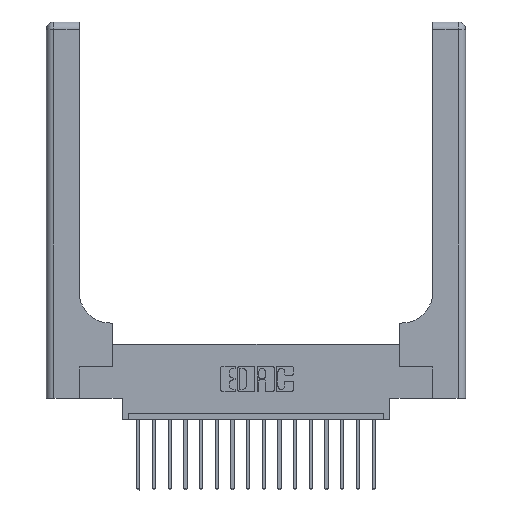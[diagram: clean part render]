
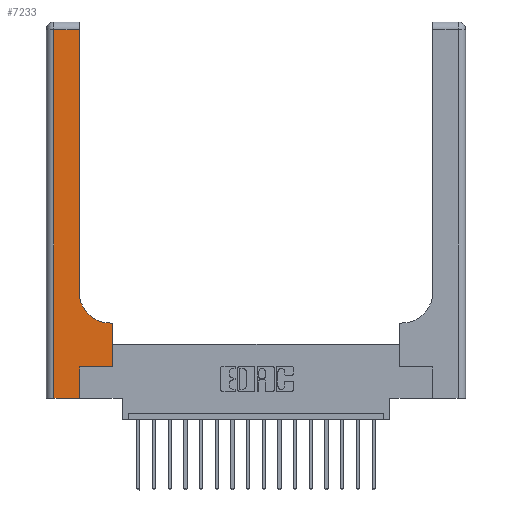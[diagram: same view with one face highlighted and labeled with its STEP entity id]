
A CAD part, top view. The second image highlights one B-rep face of the part: STEP entity #7233.
In plain terms, the highlighted planar face has unit normal (0, 0, 1).
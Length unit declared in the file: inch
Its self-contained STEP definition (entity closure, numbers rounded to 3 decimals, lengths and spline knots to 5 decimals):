
#9 = CARTESIAN_POINT ( 'NONE',  ( 0.06, 3., 0.37 ) ) ;
#205 = LINE ( 'NONE', #4086, #1102 ) ;
#412 = ORIENTED_EDGE ( 'NONE', *, *, #15414, .T. ) ;
#486 = DIRECTION ( 'NONE',  ( -1., 0., 0. ) ) ;
#812 = VECTOR ( 'NONE', #4106, 39.37008 ) ;
#978 = EDGE_LOOP ( 'NONE', ( #1641, #412, #14996, #4080, #8999, #10588, #2637, #17993, #13572 ) ) ;
#985 = CARTESIAN_POINT ( 'NONE',  ( 0., 2.94, 0.37 ) ) ;
#1102 = VECTOR ( 'NONE', #8644, 39.37008 ) ;
#1524 = CARTESIAN_POINT ( 'NONE',  ( 0., 0., 0.37 ) ) ;
#1550 = VECTOR ( 'NONE', #486, 39.37008 ) ;
#1641 = ORIENTED_EDGE ( 'NONE', *, *, #18540, .T. ) ;
#1730 = VERTEX_POINT ( 'NONE', #8140 ) ;
#2637 = ORIENTED_EDGE ( 'NONE', *, *, #5337, .T. ) ;
#2975 = VECTOR ( 'NONE', #3086, 39.37008 ) ;
#3002 = VECTOR ( 'NONE', #10304, 39.37008 ) ;
#3086 = DIRECTION ( 'NONE',  ( 0., -1., 0. ) ) ;
#3801 = DIRECTION ( 'NONE',  ( -1., 0., 0. ) ) ;
#3985 = CARTESIAN_POINT ( 'NONE',  ( 0.51, 0.6, 0.37 ) ) ;
#4080 = ORIENTED_EDGE ( 'NONE', *, *, #17657, .T. ) ;
#4086 = CARTESIAN_POINT ( 'NONE',  ( 0.26, 3., 0.37 ) ) ;
#4106 = DIRECTION ( 'NONE',  ( 1., 0., 0. ) ) ;
#4174 = LINE ( 'NONE', #18143, #18634 ) ;
#5337 = EDGE_CURVE ( 'NONE', #13479, #11984, #10361, .T. ) ;
#5340 = DIRECTION ( 'NONE',  ( 1., 0., 0. ) ) ;
#5829 = VECTOR ( 'NONE', #3801, 39.37008 ) ;
#6020 = CARTESIAN_POINT ( 'NONE',  ( 0.26, 2.94, 0.37 ) ) ;
#6306 = LINE ( 'NONE', #8536, #812 ) ;
#6322 = LINE ( 'NONE', #12239, #1550 ) ;
#6421 = VERTEX_POINT ( 'NONE', #3985 ) ;
#6530 = DIRECTION ( 'NONE',  ( 0., 0., -1. ) ) ;
#6581 = VERTEX_POINT ( 'NONE', #17558 ) ;
#6830 = LINE ( 'NONE', #9, #2975 ) ;
#7233 = ADVANCED_FACE ( 'NONE', ( #8741 ), #17638, .F. ) ;
#8039 = CARTESIAN_POINT ( 'NONE',  ( 0., 3., 0.37 ) ) ;
#8140 = CARTESIAN_POINT ( 'NONE',  ( 0.265, 0., 0.37 ) ) ;
#8175 = CIRCLE ( 'NONE', #14443, 0.25 ) ;
#8536 = CARTESIAN_POINT ( 'NONE',  ( 0.265, 0.25, 0.37 ) ) ;
#8644 = DIRECTION ( 'NONE',  ( 0., 1., 0. ) ) ;
#8741 = FACE_OUTER_BOUND ( 'NONE', #978, .T. ) ;
#8908 = AXIS2_PLACEMENT_3D ( 'NONE', #8039, #9368, #10792 ) ;
#8999 = ORIENTED_EDGE ( 'NONE', *, *, #17158, .T. ) ;
#9368 = DIRECTION ( 'NONE',  ( 0., 0., -1. ) ) ;
#9685 = LINE ( 'NONE', #985, #5829 ) ;
#9704 = VECTOR ( 'NONE', #17058, 39.37008 ) ;
#10067 = CARTESIAN_POINT ( 'NONE',  ( 0.265, 0.25, 0.37 ) ) ;
#10304 = DIRECTION ( 'NONE',  ( 1., 0., 0. ) ) ;
#10361 = LINE ( 'NONE', #12723, #9704 ) ;
#10588 = ORIENTED_EDGE ( 'NONE', *, *, #13125, .T. ) ;
#10792 = DIRECTION ( 'NONE',  ( -1., 0., 0. ) ) ;
#10891 = DIRECTION ( 'NONE',  ( 0., 1., 0. ) ) ;
#11281 = VERTEX_POINT ( 'NONE', #18059 ) ;
#11462 = CARTESIAN_POINT ( 'NONE',  ( 0.06, 2.94, 0.37 ) ) ;
#11984 = VERTEX_POINT ( 'NONE', #15474 ) ;
#12239 = CARTESIAN_POINT ( 'NONE',  ( 0.26, 0.6, 0.37 ) ) ;
#12521 = EDGE_CURVE ( 'NONE', #6421, #11281, #8175, .T. ) ;
#12723 = CARTESIAN_POINT ( 'NONE',  ( 0.528, 0.25, 0.37 ) ) ;
#12726 = EDGE_CURVE ( 'NONE', #11984, #6421, #6322, .T. ) ;
#13125 = EDGE_CURVE ( 'NONE', #14306, #13479, #6306, .T. ) ;
#13479 = VERTEX_POINT ( 'NONE', #16935 ) ;
#13572 = ORIENTED_EDGE ( 'NONE', *, *, #12521, .T. ) ;
#13788 = CARTESIAN_POINT ( 'NONE',  ( 0.51, 0.85, 0.37 ) ) ;
#14306 = VERTEX_POINT ( 'NONE', #10067 ) ;
#14443 = AXIS2_PLACEMENT_3D ( 'NONE', #13788, #6530, #5340 ) ;
#14996 = ORIENTED_EDGE ( 'NONE', *, *, #18241, .T. ) ;
#15414 = EDGE_CURVE ( 'NONE', #15653, #16050, #9685, .T. ) ;
#15474 = CARTESIAN_POINT ( 'NONE',  ( 0.528, 0.6, 0.37 ) ) ;
#15653 = VERTEX_POINT ( 'NONE', #6020 ) ;
#15962 = LINE ( 'NONE', #1524, #3002 ) ;
#16050 = VERTEX_POINT ( 'NONE', #11462 ) ;
#16935 = CARTESIAN_POINT ( 'NONE',  ( 0.528, 0.25, 0.37 ) ) ;
#17058 = DIRECTION ( 'NONE',  ( 0., 1., 0. ) ) ;
#17158 = EDGE_CURVE ( 'NONE', #1730, #14306, #4174, .T. ) ;
#17558 = CARTESIAN_POINT ( 'NONE',  ( 0.06, 0., 0.37 ) ) ;
#17638 = PLANE ( 'NONE',  #8908 ) ;
#17657 = EDGE_CURVE ( 'NONE', #6581, #1730, #15962, .T. ) ;
#17993 = ORIENTED_EDGE ( 'NONE', *, *, #12726, .T. ) ;
#18059 = CARTESIAN_POINT ( 'NONE',  ( 0.26, 0.85, 0.37 ) ) ;
#18143 = CARTESIAN_POINT ( 'NONE',  ( 0.265, 0., 0.37 ) ) ;
#18241 = EDGE_CURVE ( 'NONE', #16050, #6581, #6830, .T. ) ;
#18540 = EDGE_CURVE ( 'NONE', #11281, #15653, #205, .T. ) ;
#18634 = VECTOR ( 'NONE', #10891, 39.37008 ) ;
